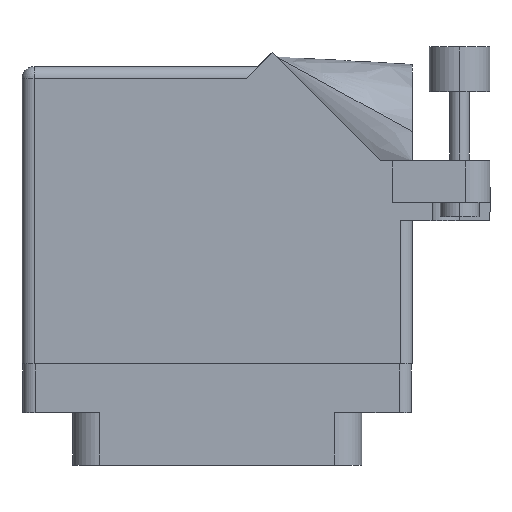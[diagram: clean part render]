
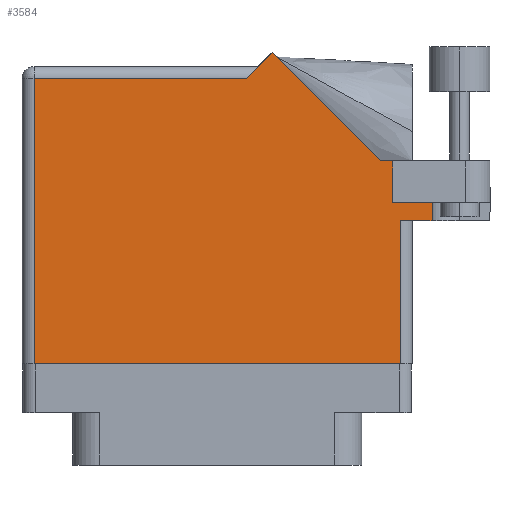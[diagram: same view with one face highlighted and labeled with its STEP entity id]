
A CAD part, front view. The second image highlights one B-rep face of the part: STEP entity #3584.
In plain terms, the highlighted face is planar.
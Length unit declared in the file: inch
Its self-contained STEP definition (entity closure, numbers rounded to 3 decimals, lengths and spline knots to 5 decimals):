
#1590 = VECTOR ( 'NONE', #7817, 39.37008 ) ;
#1644 = DIRECTION ( 'NONE',  ( -0.707, -0.707, 0. ) ) ;
#1727 = VECTOR ( 'NONE', #37698, 39.37008 ) ;
#1874 = ORIENTED_EDGE ( 'NONE', *, *, #34062, .T. ) ;
#2047 = DIRECTION ( 'NONE',  ( 0., -1., 0. ) ) ;
#2093 = CARTESIAN_POINT ( 'NONE',  ( 0.905, 0.731, 0.455 ) ) ;
#2389 = ORIENTED_EDGE ( 'NONE', *, *, #7448, .F. ) ;
#2747 = AXIS2_PLACEMENT_3D ( 'NONE', #18709, #10398, #15864 ) ;
#2842 = ORIENTED_EDGE ( 'NONE', *, *, #22469, .T. ) ;
#3121 = VECTOR ( 'NONE', #31168, 39.37008 ) ;
#3190 = EDGE_CURVE ( 'NONE', #24799, #23924, #4968, .T. ) ;
#3409 = VERTEX_POINT ( 'NONE', #21303 ) ;
#3584 = ADVANCED_FACE ( 'NONE', ( #11288 ), #9574, .F. ) ;
#3950 = VERTEX_POINT ( 'NONE', #6225 ) ;
#4074 = CARTESIAN_POINT ( 'NONE',  ( 1.1065, 0.637, 0.455 ) ) ;
#4085 = CARTESIAN_POINT ( 'NONE',  ( -0.943, 1.368, 0.455 ) ) ;
#4968 = LINE ( 'NONE', #29652, #8910 ) ;
#5207 = LINE ( 'NONE', #17928, #25277 ) ;
#5446 = ORIENTED_EDGE ( 'NONE', *, *, #16093, .F. ) ;
#6225 = CARTESIAN_POINT ( 'NONE',  ( -0.943, -0.1, 0.455 ) ) ;
#6941 = LINE ( 'NONE', #33173, #1590 ) ;
#7448 = EDGE_CURVE ( 'NONE', #24799, #38983, #32908, .T. ) ;
#7817 = DIRECTION ( 'NONE',  ( -0.707, 0.707, 0. ) ) ;
#8155 = EDGE_CURVE ( 'NONE', #37527, #20245, #6941, .T. ) ;
#8656 = CARTESIAN_POINT ( 'NONE',  ( 0.905, 0.731, 0.455 ) ) ;
#8910 = VECTOR ( 'NONE', #38649, 39.37008 ) ;
#9574 = PLANE ( 'NONE',  #2747 ) ;
#10398 = DIRECTION ( 'NONE',  ( 0., 0., -1. ) ) ;
#10535 = CARTESIAN_POINT ( 'NONE',  ( 0.943, 0.637, 0.455 ) ) ;
#10905 = VERTEX_POINT ( 'NONE', #4085 ) ;
#11288 = FACE_OUTER_BOUND ( 'NONE', #27059, .T. ) ;
#11468 = VECTOR ( 'NONE', #1644, 39.37008 ) ;
#11720 = VECTOR ( 'NONE', #17054, 39.37008 ) ;
#12241 = CARTESIAN_POINT ( 'NONE',  ( 0.943, 0.637, 0.455 ) ) ;
#12742 = ORIENTED_EDGE ( 'NONE', *, *, #18713, .T. ) ;
#13754 = VERTEX_POINT ( 'NONE', #4074 ) ;
#13948 = LINE ( 'NONE', #26747, #11468 ) ;
#14077 = DIRECTION ( 'NONE',  ( 0., -1., 0. ) ) ;
#15667 = VECTOR ( 'NONE', #14077, 39.37008 ) ;
#15864 = DIRECTION ( 'NONE',  ( -1., 0., 0. ) ) ;
#16093 = EDGE_CURVE ( 'NONE', #38983, #13754, #27872, .T. ) ;
#17054 = DIRECTION ( 'NONE',  ( 1., 0., 0. ) ) ;
#17135 = CARTESIAN_POINT ( 'NONE',  ( 1.405, 0.944, 0.455 ) ) ;
#17928 = CARTESIAN_POINT ( 'NONE',  ( -0.943, -0.1, 0.455 ) ) ;
#18709 = CARTESIAN_POINT ( 'NONE',  ( -1.005, 1.43, 0.455 ) ) ;
#18713 = EDGE_CURVE ( 'NONE', #40194, #22727, #37383, .T. ) ;
#18766 = DIRECTION ( 'NONE',  ( 0., 1., 0. ) ) ;
#19589 = ORIENTED_EDGE ( 'NONE', *, *, #29931, .T. ) ;
#19801 = LINE ( 'NONE', #22118, #1727 ) ;
#20077 = ORIENTED_EDGE ( 'NONE', *, *, #8155, .T. ) ;
#20245 = VERTEX_POINT ( 'NONE', #29684 ) ;
#20909 = EDGE_CURVE ( 'NONE', #23924, #37527, #26315, .T. ) ;
#21303 = CARTESIAN_POINT ( 'NONE',  ( 0.15, 1.368, 0.455 ) ) ;
#21659 = EDGE_CURVE ( 'NONE', #10905, #3950, #5207, .T. ) ;
#21745 = ORIENTED_EDGE ( 'NONE', *, *, #3190, .T. ) ;
#22118 = CARTESIAN_POINT ( 'NONE',  ( -1.005, 1.368, 0.455 ) ) ;
#22469 = EDGE_CURVE ( 'NONE', #3409, #10905, #19801, .T. ) ;
#22579 = ORIENTED_EDGE ( 'NONE', *, *, #20909, .T. ) ;
#22727 = VERTEX_POINT ( 'NONE', #10535 ) ;
#23016 = CARTESIAN_POINT ( 'NONE',  ( 1.1065, 1.06177, 0.455 ) ) ;
#23672 = VECTOR ( 'NONE', #18766, 39.37008 ) ;
#23924 = VERTEX_POINT ( 'NONE', #38446 ) ;
#24799 = VERTEX_POINT ( 'NONE', #8656 ) ;
#25277 = VECTOR ( 'NONE', #2047, 39.37008 ) ;
#26315 = LINE ( 'NONE', #17135, #37054 ) ;
#26747 = CARTESIAN_POINT ( 'NONE',  ( 0.212, 1.43, 0.455 ) ) ;
#27059 = EDGE_LOOP ( 'NONE', ( #19589, #12742, #1874, #5446, #2389, #21745, #22579, #20077, #31889, #2842, #36074 ) ) ;
#27872 = LINE ( 'NONE', #23016, #15667 ) ;
#28302 = LINE ( 'NONE', #31179, #28759 ) ;
#28432 = DIRECTION ( 'NONE',  ( 1., 0., 0. ) ) ;
#28759 = VECTOR ( 'NONE', #28432, 39.37008 ) ;
#29652 = CARTESIAN_POINT ( 'NONE',  ( 0.905, 0.731, 0.455 ) ) ;
#29684 = CARTESIAN_POINT ( 'NONE',  ( 0.28271, 1.50071, 0.455 ) ) ;
#29931 = EDGE_CURVE ( 'NONE', #3950, #40194, #32253, .T. ) ;
#31168 = DIRECTION ( 'NONE',  ( 1., 0., 0. ) ) ;
#31179 = CARTESIAN_POINT ( 'NONE',  ( 1.005, 0.637, 0.455 ) ) ;
#31212 = CARTESIAN_POINT ( 'NONE',  ( 1.1065, 0.731, 0.455 ) ) ;
#31731 = EDGE_CURVE ( 'NONE', #20245, #3409, #13948, .T. ) ;
#31804 = CARTESIAN_POINT ( 'NONE',  ( 0.943, -0.1, 0.455 ) ) ;
#31889 = ORIENTED_EDGE ( 'NONE', *, *, #31731, .T. ) ;
#32253 = LINE ( 'NONE', #35703, #11720 ) ;
#32908 = LINE ( 'NONE', #2093, #3121 ) ;
#33173 = CARTESIAN_POINT ( 'NONE',  ( 0.83942, 0.944, 0.455 ) ) ;
#33284 = CARTESIAN_POINT ( 'NONE',  ( 0.83942, 0.944, 0.455 ) ) ;
#34062 = EDGE_CURVE ( 'NONE', #22727, #13754, #28302, .T. ) ;
#35703 = CARTESIAN_POINT ( 'NONE',  ( -1.005, -0.1, 0.455 ) ) ;
#36074 = ORIENTED_EDGE ( 'NONE', *, *, #21659, .T. ) ;
#37054 = VECTOR ( 'NONE', #39450, 39.37008 ) ;
#37383 = LINE ( 'NONE', #12241, #23672 ) ;
#37527 = VERTEX_POINT ( 'NONE', #33284 ) ;
#37698 = DIRECTION ( 'NONE',  ( -1., 0., 0. ) ) ;
#38446 = CARTESIAN_POINT ( 'NONE',  ( 0.905, 0.944, 0.455 ) ) ;
#38649 = DIRECTION ( 'NONE',  ( 0., 1., 0. ) ) ;
#38983 = VERTEX_POINT ( 'NONE', #31212 ) ;
#39450 = DIRECTION ( 'NONE',  ( -1., 0., 0. ) ) ;
#40194 = VERTEX_POINT ( 'NONE', #31804 ) ;
